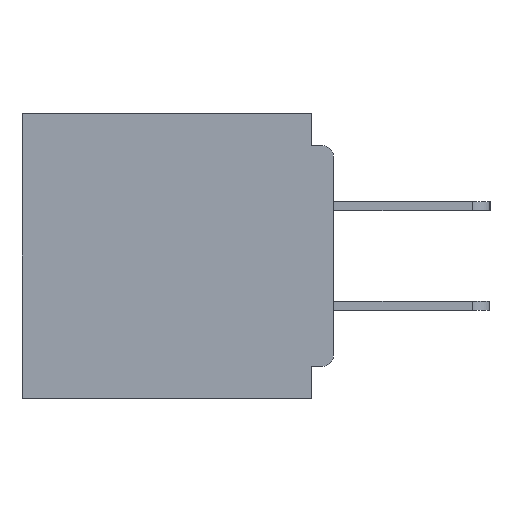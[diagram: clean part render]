
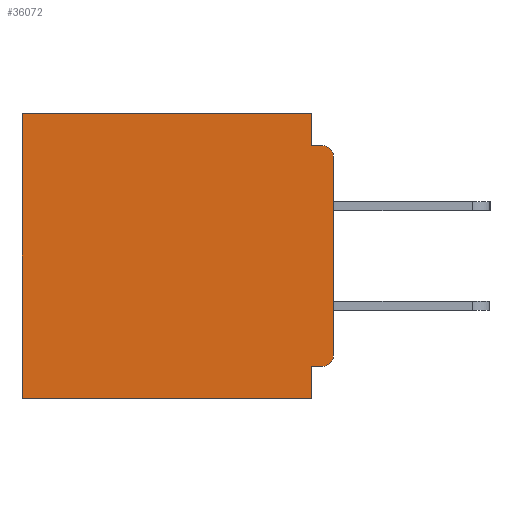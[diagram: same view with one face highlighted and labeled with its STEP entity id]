
A CAD part, left-side view. The second image highlights one B-rep face of the part: STEP entity #36072.
In plain terms, the highlighted planar face has unit normal (-1, 0, 0).
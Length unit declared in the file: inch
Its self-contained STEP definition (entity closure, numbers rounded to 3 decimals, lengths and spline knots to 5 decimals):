
#207 = VERTEX_POINT ( 'NONE', #28849 ) ;
#712 = DIRECTION ( 'NONE',  ( 0., 0., -1. ) ) ;
#857 = ORIENTED_EDGE ( 'NONE', *, *, #16604, .F. ) ;
#982 = CARTESIAN_POINT ( 'NONE',  ( 0.3, 0., -0.4 ) ) ;
#1124 = LINE ( 'NONE', #12455, #41130 ) ;
#1261 = PLANE ( 'NONE',  #35180 ) ;
#1598 = CARTESIAN_POINT ( 'NONE',  ( 0.3, 0., -0.355 ) ) ;
#2770 = DIRECTION ( 'NONE',  ( 0., 0., -1. ) ) ;
#3395 = ORIENTED_EDGE ( 'NONE', *, *, #40623, .F. ) ;
#4267 = VECTOR ( 'NONE', #10088, 39.37008 ) ;
#4478 = VERTEX_POINT ( 'NONE', #40472 ) ;
#4547 = DIRECTION ( 'NONE',  ( 0., 0., -1. ) ) ;
#5274 = CARTESIAN_POINT ( 'NONE',  ( 0.3, 0.015, -0.355 ) ) ;
#5286 = LINE ( 'NONE', #23010, #4267 ) ;
#5429 = ORIENTED_EDGE ( 'NONE', *, *, #25929, .F. ) ;
#5565 = CARTESIAN_POINT ( 'NONE',  ( 0.3, 0.031, 0. ) ) ;
#6076 = LINE ( 'NONE', #18300, #39466 ) ;
#6559 = DIRECTION ( 'NONE',  ( 0., 1., 0. ) ) ;
#6868 = DIRECTION ( 'NONE',  ( 0., 0., -1. ) ) ;
#7810 = VERTEX_POINT ( 'NONE', #17052 ) ;
#9074 = VERTEX_POINT ( 'NONE', #27987 ) ;
#9093 = VERTEX_POINT ( 'NONE', #5274 ) ;
#9188 = DIRECTION ( 'NONE',  ( 0., -1., 0. ) ) ;
#9414 = DIRECTION ( 'NONE',  ( 0., 0., -1. ) ) ;
#9810 = ORIENTED_EDGE ( 'NONE', *, *, #25848, .F. ) ;
#9832 = ORIENTED_EDGE ( 'NONE', *, *, #12294, .T. ) ;
#10088 = DIRECTION ( 'NONE',  ( 0., 0., -1. ) ) ;
#12224 = CIRCLE ( 'NONE', #29580, 0.015 ) ;
#12294 = EDGE_CURVE ( 'NONE', #35643, #9074, #6076, .T. ) ;
#12455 = CARTESIAN_POINT ( 'NONE',  ( 0.3, 0., -0.4 ) ) ;
#12478 = EDGE_CURVE ( 'NONE', #9093, #207, #33454, .T. ) ;
#13733 = CARTESIAN_POINT ( 'NONE',  ( 0.3, 0.031, 0. ) ) ;
#15223 = EDGE_CURVE ( 'NONE', #33612, #25570, #5286, .T. ) ;
#16021 = CARTESIAN_POINT ( 'NONE',  ( 0.3, 0.015, -0.34 ) ) ;
#16604 = EDGE_CURVE ( 'NONE', #35643, #4478, #21384, .T. ) ;
#17052 = CARTESIAN_POINT ( 'NONE',  ( 0.3, 0.437, -0.4 ) ) ;
#17243 = ORIENTED_EDGE ( 'NONE', *, *, #27637, .T. ) ;
#18046 = EDGE_CURVE ( 'NONE', #9074, #7810, #18232, .T. ) ;
#18232 = LINE ( 'NONE', #32668, #41836 ) ;
#18300 = CARTESIAN_POINT ( 'NONE',  ( 0.3, 0., 0. ) ) ;
#18759 = AXIS2_PLACEMENT_3D ( 'NONE', #16021, #38531, #19269 ) ;
#19269 = DIRECTION ( 'NONE',  ( 0., 0., -1. ) ) ;
#21384 = LINE ( 'NONE', #13733, #37469 ) ;
#21524 = DIRECTION ( 'NONE',  ( 0., 1., 0. ) ) ;
#21560 = LINE ( 'NONE', #25349, #28096 ) ;
#22173 = CARTESIAN_POINT ( 'NONE',  ( 0.3, 0.031, -0.355 ) ) ;
#22286 = DIRECTION ( 'NONE',  ( -1., 0., 0. ) ) ;
#22526 = VERTEX_POINT ( 'NONE', #32513 ) ;
#23010 = CARTESIAN_POINT ( 'NONE',  ( 0.3, 0.031, -0.4 ) ) ;
#24024 = DIRECTION ( 'NONE',  ( 1., 0., 0. ) ) ;
#24209 = DIRECTION ( 'NONE',  ( 0., 1., 0. ) ) ;
#24493 = ORIENTED_EDGE ( 'NONE', *, *, #15223, .F. ) ;
#25349 = CARTESIAN_POINT ( 'NONE',  ( 0.3, 0., -0.045 ) ) ;
#25570 = VERTEX_POINT ( 'NONE', #30130 ) ;
#25757 = ORIENTED_EDGE ( 'NONE', *, *, #35488, .F. ) ;
#25800 = CARTESIAN_POINT ( 'NONE',  ( 0.3, 0.015, -0.045 ) ) ;
#25848 = EDGE_CURVE ( 'NONE', #22526, #207, #1124, .T. ) ;
#25929 = EDGE_CURVE ( 'NONE', #25570, #7810, #30602, .T. ) ;
#27637 = EDGE_CURVE ( 'NONE', #22526, #32210, #12224, .T. ) ;
#27987 = CARTESIAN_POINT ( 'NONE',  ( 0.3, 0.437, 0. ) ) ;
#28096 = VECTOR ( 'NONE', #9188, 39.37008 ) ;
#28849 = CARTESIAN_POINT ( 'NONE',  ( 0.3, 0., -0.34 ) ) ;
#29275 = CARTESIAN_POINT ( 'NONE',  ( 0.3, 0., -0.4 ) ) ;
#29580 = AXIS2_PLACEMENT_3D ( 'NONE', #41532, #22286, #2770 ) ;
#30130 = CARTESIAN_POINT ( 'NONE',  ( 0.3, 0.031, -0.4 ) ) ;
#30602 = LINE ( 'NONE', #29275, #38137 ) ;
#32210 = VERTEX_POINT ( 'NONE', #25800 ) ;
#32513 = CARTESIAN_POINT ( 'NONE',  ( 0.3, 0., -0.06 ) ) ;
#32668 = CARTESIAN_POINT ( 'NONE',  ( 0.3, 0.437, -0.4 ) ) ;
#33065 = ORIENTED_EDGE ( 'NONE', *, *, #18046, .T. ) ;
#33454 = CIRCLE ( 'NONE', #18759, 0.015 ) ;
#33612 = VERTEX_POINT ( 'NONE', #22173 ) ;
#35180 = AXIS2_PLACEMENT_3D ( 'NONE', #982, #24024, #4547 ) ;
#35488 = EDGE_CURVE ( 'NONE', #9093, #33612, #36578, .T. ) ;
#35582 = VECTOR ( 'NONE', #24209, 39.37008 ) ;
#35643 = VERTEX_POINT ( 'NONE', #5565 ) ;
#36072 = ADVANCED_FACE ( 'NONE', ( #38022 ), #1261, .F. ) ;
#36578 = LINE ( 'NONE', #1598, #35582 ) ;
#37120 = EDGE_LOOP ( 'NONE', ( #9810, #17243, #3395, #857, #9832, #33065, #5429, #24493, #25757, #39199 ) ) ;
#37469 = VECTOR ( 'NONE', #712, 39.37008 ) ;
#38022 = FACE_OUTER_BOUND ( 'NONE', #37120, .T. ) ;
#38137 = VECTOR ( 'NONE', #6559, 39.37008 ) ;
#38531 = DIRECTION ( 'NONE',  ( -1., 0., 0. ) ) ;
#39199 = ORIENTED_EDGE ( 'NONE', *, *, #12478, .T. ) ;
#39466 = VECTOR ( 'NONE', #21524, 39.37008 ) ;
#40472 = CARTESIAN_POINT ( 'NONE',  ( 0.3, 0.031, -0.045 ) ) ;
#40623 = EDGE_CURVE ( 'NONE', #4478, #32210, #21560, .T. ) ;
#41130 = VECTOR ( 'NONE', #9414, 39.37008 ) ;
#41532 = CARTESIAN_POINT ( 'NONE',  ( 0.3, 0.015, -0.06 ) ) ;
#41836 = VECTOR ( 'NONE', #6868, 39.37008 ) ;
